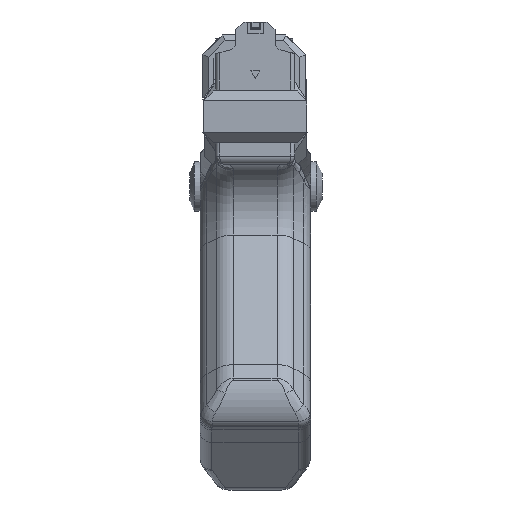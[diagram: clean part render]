
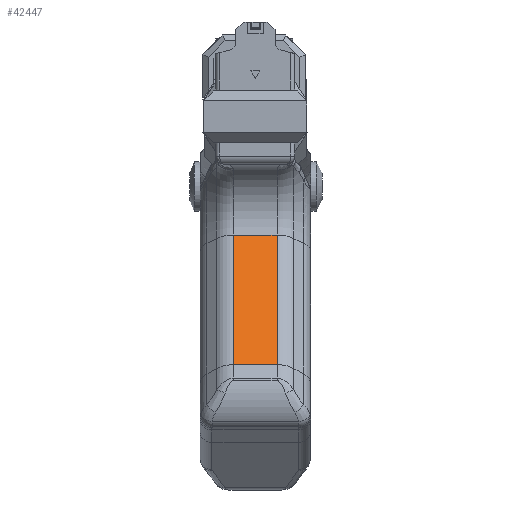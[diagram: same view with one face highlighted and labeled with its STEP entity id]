
A CAD part, front view. The second image highlights one B-rep face of the part: STEP entity #42447.
In plain terms, the highlighted face is planar.
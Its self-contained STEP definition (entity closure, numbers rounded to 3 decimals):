
#3829=LINE('',#111674,#7730);
#3841=LINE('',#111714,#7742);
#3842=LINE('',#111717,#7743);
#3843=LINE('',#111718,#7744);
#7730=VECTOR('',#52337,10.);
#7742=VECTOR('',#52373,10.);
#7743=VECTOR('',#52376,10.);
#7744=VECTOR('',#52377,10.);
#9763=PLANE('',#45177);
#11469=FACE_OUTER_BOUND('',#13778,.T.);
#13778=EDGE_LOOP('',(#35926,#35927,#35928,#35929));
#19901=VERTEX_POINT('',#110642);
#19956=VERTEX_POINT('',#111673);
#19964=VERTEX_POINT('',#111712);
#19965=VERTEX_POINT('',#111716);
#25571=EDGE_CURVE('',#19901,#19956,#3829,.T.);
#25587=EDGE_CURVE('',#19901,#19964,#3841,.T.);
#25588=EDGE_CURVE('',#19964,#19965,#3842,.T.);
#25589=EDGE_CURVE('',#19965,#19956,#3843,.T.);
#35926=ORIENTED_EDGE('',*,*,#25587,.T.);
#35927=ORIENTED_EDGE('',*,*,#25588,.T.);
#35928=ORIENTED_EDGE('',*,*,#25589,.T.);
#35929=ORIENTED_EDGE('',*,*,#25571,.F.);
#42447=ADVANCED_FACE('',(#11469),#9763,.F.);
#45177=AXIS2_PLACEMENT_3D('',#111715,#52374,#52375);
#52337=DIRECTION('',(0.,-0.84,0.543));
#52373=DIRECTION('',(-1.,0.,0.));
#52374=DIRECTION('center_axis',(0.,-0.543,-0.84));
#52375=DIRECTION('ref_axis',(0.,-0.84,0.543));
#52376=DIRECTION('',(0.,-0.84,0.543));
#52377=DIRECTION('',(1.,0.,0.));
#110642=CARTESIAN_POINT('',(5.515,-30.,115.));
#111673=CARTESIAN_POINT('',(5.515,-62.78,136.201));
#111674=CARTESIAN_POINT('',(5.515,-25.665,112.196));
#111712=CARTESIAN_POINT('',(-5.515,-30.,115.));
#111714=CARTESIAN_POINT('',(4.,-30.,115.));
#111715=CARTESIAN_POINT('Origin',(14.,-30.,115.));
#111716=CARTESIAN_POINT('',(-5.515,-62.78,136.201));
#111717=CARTESIAN_POINT('',(-5.515,-25.665,112.196));
#111718=CARTESIAN_POINT('',(14.,-62.78,136.201));
